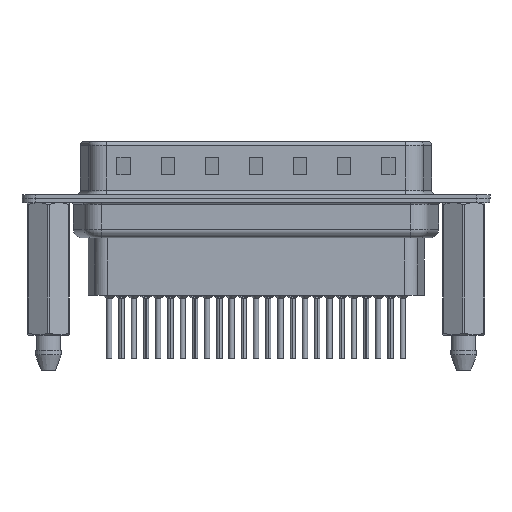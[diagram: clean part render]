
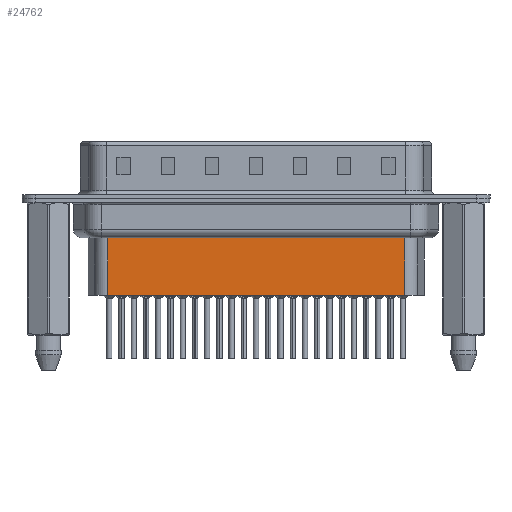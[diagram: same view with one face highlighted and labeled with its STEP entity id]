
A CAD part, front view. The second image highlights one B-rep face of the part: STEP entity #24762.
In plain terms, the highlighted planar face has unit normal (0, -1, 0).
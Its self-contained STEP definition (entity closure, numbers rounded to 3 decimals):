
#95 = EDGE_CURVE ( 'NONE', #2136, #5336, #21027, .T. ) ;
#126 = DIRECTION ( 'NONE',  ( 0., 0., -1. ) ) ;
#619 = EDGE_CURVE ( 'NONE', #5724, #5713, #10975, .T. ) ;
#1833 = PLANE ( 'NONE',  #2949 ) ;
#2046 = CARTESIAN_POINT ( 'NONE',  ( 6.459, -3.5, -4.097 ) ) ;
#2136 = VERTEX_POINT ( 'NONE', #6632 ) ;
#2164 = VECTOR ( 'NONE', #8669, 1000. ) ;
#2949 = AXIS2_PLACEMENT_3D ( 'NONE', #19016, #25630, #8311 ) ;
#3094 = ORIENTED_EDGE ( 'NONE', *, *, #16489, .T. ) ;
#3698 = DIRECTION ( 'NONE',  ( 0., 0., -1. ) ) ;
#5336 = VERTEX_POINT ( 'NONE', #12714 ) ;
#5398 = CARTESIAN_POINT ( 'NONE',  ( 6.706, -3.5, -10.95 ) ) ;
#5713 = VERTEX_POINT ( 'NONE', #10575 ) ;
#5724 = VERTEX_POINT ( 'NONE', #23529 ) ;
#6619 = CARTESIAN_POINT ( 'NONE',  ( 40.344, -3.5, -3.1 ) ) ;
#6628 = FACE_OUTER_BOUND ( 'NONE', #26671, .T. ) ;
#6632 = CARTESIAN_POINT ( 'NONE',  ( 6.706, -3.5, -4.097 ) ) ;
#7169 = VECTOR ( 'NONE', #10030, 1000. ) ;
#8311 = DIRECTION ( 'NONE',  ( 1., 0., 0. ) ) ;
#8669 = DIRECTION ( 'NONE',  ( -1., 0., 0. ) ) ;
#10030 = DIRECTION ( 'NONE',  ( -1., 0., 0. ) ) ;
#10575 = CARTESIAN_POINT ( 'NONE',  ( 40.344, -3.5, -10.95 ) ) ;
#10649 = LINE ( 'NONE', #2046, #2164 ) ;
#10975 = LINE ( 'NONE', #6619, #16776 ) ;
#12690 = ORIENTED_EDGE ( 'NONE', *, *, #19381, .F. ) ;
#12714 = CARTESIAN_POINT ( 'NONE',  ( 6.706, -3.5, -10.95 ) ) ;
#13002 = ORIENTED_EDGE ( 'NONE', *, *, #95, .T. ) ;
#14401 = LINE ( 'NONE', #5398, #7169 ) ;
#16489 = EDGE_CURVE ( 'NONE', #5724, #2136, #10649, .T. ) ;
#16680 = VECTOR ( 'NONE', #3698, 1000. ) ;
#16776 = VECTOR ( 'NONE', #126, 1000. ) ;
#19016 = CARTESIAN_POINT ( 'NONE',  ( 6.706, -3.5, -3.1 ) ) ;
#19188 = CARTESIAN_POINT ( 'NONE',  ( 6.706, -3.5, -3.1 ) ) ;
#19381 = EDGE_CURVE ( 'NONE', #5713, #5336, #14401, .T. ) ;
#20489 = ORIENTED_EDGE ( 'NONE', *, *, #619, .F. ) ;
#21027 = LINE ( 'NONE', #19188, #16680 ) ;
#23529 = CARTESIAN_POINT ( 'NONE',  ( 40.344, -3.5, -4.097 ) ) ;
#24762 = ADVANCED_FACE ( 'NONE', ( #6628 ), #1833, .T. ) ;
#25630 = DIRECTION ( 'NONE',  ( 0., -1., 0. ) ) ;
#26671 = EDGE_LOOP ( 'NONE', ( #20489, #3094, #13002, #12690 ) ) ;
